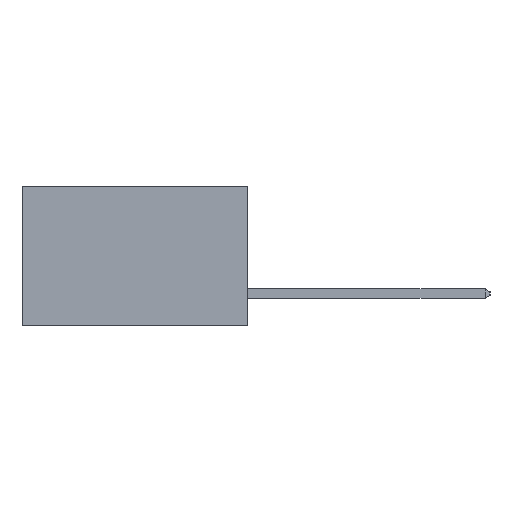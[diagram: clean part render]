
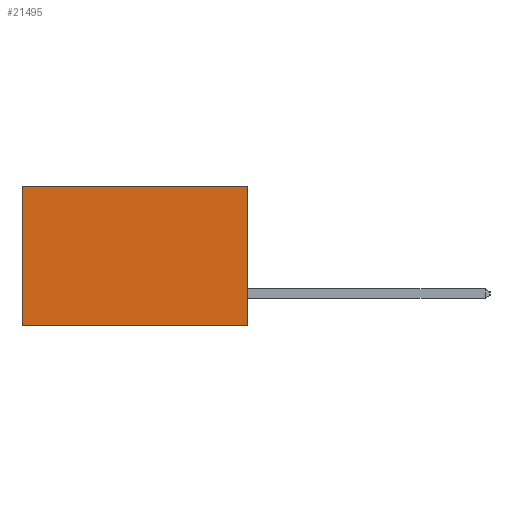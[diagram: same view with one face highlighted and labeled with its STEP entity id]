
A CAD part, left-side view. The second image highlights one B-rep face of the part: STEP entity #21495.
In plain terms, the highlighted planar face has unit normal (-1, 0, 0).
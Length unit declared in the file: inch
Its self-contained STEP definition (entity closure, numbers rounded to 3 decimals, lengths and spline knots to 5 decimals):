
#593 = CARTESIAN_POINT ( 'NONE',  ( 0.298, 0., -0.37 ) ) ;
#677 = ORIENTED_EDGE ( 'NONE', *, *, #15373, .F. ) ;
#1081 = VERTEX_POINT ( 'NONE', #4947 ) ;
#2130 = VERTEX_POINT ( 'NONE', #9109 ) ;
#4383 = VERTEX_POINT ( 'NONE', #593 ) ;
#4663 = DIRECTION ( 'NONE',  ( 0., 0., -1. ) ) ;
#4947 = CARTESIAN_POINT ( 'NONE',  ( 0.298, 0.6, 0. ) ) ;
#5257 = DIRECTION ( 'NONE',  ( 0., 0., -1. ) ) ;
#6214 = ORIENTED_EDGE ( 'NONE', *, *, #19812, .F. ) ;
#6868 = EDGE_CURVE ( 'NONE', #1081, #25819, #23104, .T. ) ;
#8095 = DIRECTION ( 'NONE',  ( 0., 1., 0. ) ) ;
#8180 = VECTOR ( 'NONE', #8095, 39.37008 ) ;
#9109 = CARTESIAN_POINT ( 'NONE',  ( 0.298, 0., 0. ) ) ;
#10184 = VECTOR ( 'NONE', #18665, 39.37008 ) ;
#10465 = AXIS2_PLACEMENT_3D ( 'NONE', #24216, #18058, #5257 ) ;
#11618 = PLANE ( 'NONE',  #10465 ) ;
#13201 = CARTESIAN_POINT ( 'NONE',  ( 0.298, 0.6, 0. ) ) ;
#14712 = EDGE_CURVE ( 'NONE', #2130, #1081, #20130, .T. ) ;
#15373 = EDGE_CURVE ( 'NONE', #4383, #25819, #24914, .T. ) ;
#16006 = ORIENTED_EDGE ( 'NONE', *, *, #6868, .T. ) ;
#16931 = VECTOR ( 'NONE', #4663, 39.37008 ) ;
#17357 = FACE_OUTER_BOUND ( 'NONE', #18930, .T. ) ;
#18058 = DIRECTION ( 'NONE',  ( 1., 0., 0. ) ) ;
#18665 = DIRECTION ( 'NONE',  ( 0., 0., -1. ) ) ;
#18822 = DIRECTION ( 'NONE',  ( 0., 1., 0. ) ) ;
#18930 = EDGE_LOOP ( 'NONE', ( #16006, #677, #6214, #26475 ) ) ;
#19812 = EDGE_CURVE ( 'NONE', #2130, #4383, #26875, .T. ) ;
#20130 = LINE ( 'NONE', #26860, #8180 ) ;
#21495 = ADVANCED_FACE ( 'NONE', ( #17357 ), #11618, .F. ) ;
#22845 = CARTESIAN_POINT ( 'NONE',  ( 0.298, 0., 0. ) ) ;
#23104 = LINE ( 'NONE', #13201, #16931 ) ;
#24216 = CARTESIAN_POINT ( 'NONE',  ( 0.298, 0., 0. ) ) ;
#24273 = VECTOR ( 'NONE', #18822, 39.37008 ) ;
#24914 = LINE ( 'NONE', #27001, #24273 ) ;
#25788 = CARTESIAN_POINT ( 'NONE',  ( 0.298, 0.6, -0.37 ) ) ;
#25819 = VERTEX_POINT ( 'NONE', #25788 ) ;
#26475 = ORIENTED_EDGE ( 'NONE', *, *, #14712, .T. ) ;
#26860 = CARTESIAN_POINT ( 'NONE',  ( 0.298, 0., 0. ) ) ;
#26875 = LINE ( 'NONE', #22845, #10184 ) ;
#27001 = CARTESIAN_POINT ( 'NONE',  ( 0.298, 0., -0.37 ) ) ;
